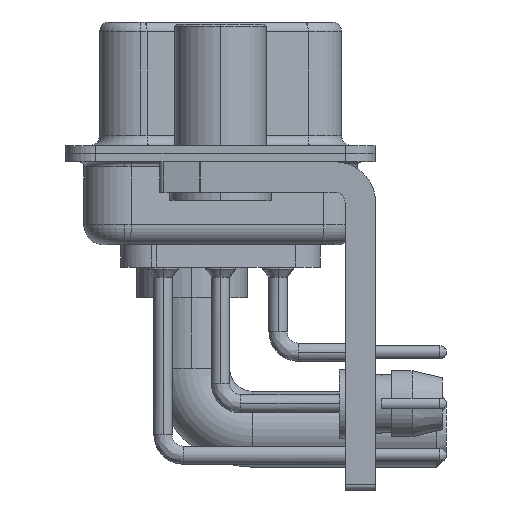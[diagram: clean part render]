
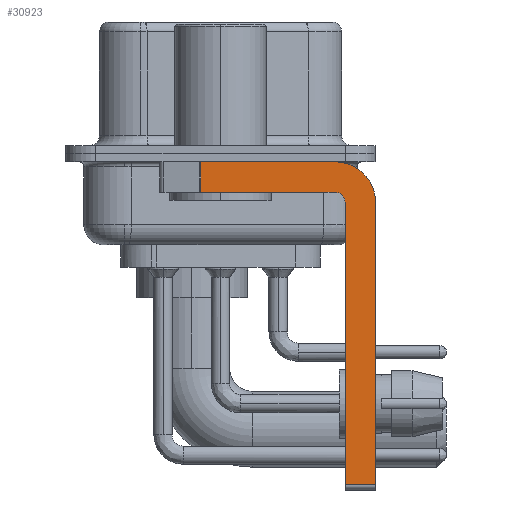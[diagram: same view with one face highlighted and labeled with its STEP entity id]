
A CAD part, left-side view. The second image highlights one B-rep face of the part: STEP entity #30923.
In plain terms, the highlighted planar face has unit normal (-1, 0, 0).
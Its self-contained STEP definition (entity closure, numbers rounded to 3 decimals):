
#96 = AXIS2_PLACEMENT_3D ( 'NONE', #14700, #20282, #21100 ) ;
#1183 = CARTESIAN_POINT ( 'NONE',  ( -2.9, 3., -0.4 ) ) ;
#1696 = VECTOR ( 'NONE', #13907, 1000. ) ;
#1845 = LINE ( 'NONE', #11345, #6708 ) ;
#3026 = DIRECTION ( 'NONE',  ( 0., 0., 1. ) ) ;
#3221 = CARTESIAN_POINT ( 'NONE',  ( -2.9, -7.65, -2.4 ) ) ;
#3273 = CARTESIAN_POINT ( 'NONE',  ( -2.9, -5.65, -2.4 ) ) ;
#3668 = ORIENTED_EDGE ( 'NONE', *, *, #4873, .T. ) ;
#4873 = EDGE_CURVE ( 'NONE', #5957, #13016, #1845, .T. ) ;
#4995 = CARTESIAN_POINT ( 'NONE',  ( -2.9, 0.978, -1.9 ) ) ;
#5515 = EDGE_CURVE ( 'NONE', #15541, #10681, #18696, .T. ) ;
#5957 = VERTEX_POINT ( 'NONE', #21525 ) ;
#6576 = EDGE_CURVE ( 'NONE', #24902, #39361, #7329, .T. ) ;
#6708 = VECTOR ( 'NONE', #36830, 1000. ) ;
#7329 = LINE ( 'NONE', #3221, #15511 ) ;
#7722 = LINE ( 'NONE', #23409, #1696 ) ;
#9892 = DIRECTION ( 'NONE',  ( 0., -1., 0. ) ) ;
#10085 = ORIENTED_EDGE ( 'NONE', *, *, #16367, .T. ) ;
#10681 = VERTEX_POINT ( 'NONE', #37434 ) ;
#11345 = CARTESIAN_POINT ( 'NONE',  ( -2.9, 0.978, -1.9 ) ) ;
#12985 = PLANE ( 'NONE',  #29920 ) ;
#13016 = VERTEX_POINT ( 'NONE', #4995 ) ;
#13907 = DIRECTION ( 'NONE',  ( 0., 1., 0. ) ) ;
#14700 = CARTESIAN_POINT ( 'NONE',  ( -2.9, -5.65, -2.4 ) ) ;
#15511 = VECTOR ( 'NONE', #15803, 1000. ) ;
#15541 = VERTEX_POINT ( 'NONE', #18514 ) ;
#15609 = ORIENTED_EDGE ( 'NONE', *, *, #5515, .F. ) ;
#15803 = DIRECTION ( 'NONE',  ( 0., 0., -1. ) ) ;
#16085 = VECTOR ( 'NONE', #3026, 1000. ) ;
#16202 = EDGE_CURVE ( 'NONE', #10681, #21532, #26743, .T. ) ;
#16367 = EDGE_CURVE ( 'NONE', #15541, #39361, #24037, .T. ) ;
#16476 = FACE_OUTER_BOUND ( 'NONE', #18847, .T. ) ;
#18172 = CARTESIAN_POINT ( 'NONE',  ( -2.9, -5.65, -0.4 ) ) ;
#18514 = CARTESIAN_POINT ( 'NONE',  ( -2.9, -6.15, -16.35 ) ) ;
#18696 = LINE ( 'NONE', #31349, #16085 ) ;
#18847 = EDGE_LOOP ( 'NONE', ( #21902, #3668, #19758, #30203, #15609, #10085, #38319, #26120 ) ) ;
#19758 = ORIENTED_EDGE ( 'NONE', *, *, #38857, .F. ) ;
#20282 = DIRECTION ( 'NONE',  ( 1., 0., 0. ) ) ;
#21100 = DIRECTION ( 'NONE',  ( 0., 0., -1. ) ) ;
#21521 = VERTEX_POINT ( 'NONE', #18172 ) ;
#21525 = CARTESIAN_POINT ( 'NONE',  ( -2.9, 0.978, -0.4 ) ) ;
#21532 = VERTEX_POINT ( 'NONE', #24800 ) ;
#21902 = ORIENTED_EDGE ( 'NONE', *, *, #35999, .F. ) ;
#22069 = AXIS2_PLACEMENT_3D ( 'NONE', #33155, #26322, #36080 ) ;
#23289 = DIRECTION ( 'NONE',  ( 0., -1., 0. ) ) ;
#23401 = VECTOR ( 'NONE', #9892, 1000. ) ;
#23409 = CARTESIAN_POINT ( 'NONE',  ( -2.9, -5.65, -1.9 ) ) ;
#23917 = EDGE_CURVE ( 'NONE', #21521, #24902, #26526, .T. ) ;
#24037 = LINE ( 'NONE', #36699, #23401 ) ;
#24800 = CARTESIAN_POINT ( 'NONE',  ( -2.9, -5.65, -1.9 ) ) ;
#24902 = VERTEX_POINT ( 'NONE', #36783 ) ;
#26120 = ORIENTED_EDGE ( 'NONE', *, *, #23917, .F. ) ;
#26279 = CARTESIAN_POINT ( 'NONE',  ( -2.9, -7.65, -16.35 ) ) ;
#26322 = DIRECTION ( 'NONE',  ( -1., 0., 0. ) ) ;
#26526 = CIRCLE ( 'NONE', #96, 2. ) ;
#26743 = CIRCLE ( 'NONE', #22069, 0.5 ) ;
#26853 = LINE ( 'NONE', #1183, #27348 ) ;
#27348 = VECTOR ( 'NONE', #23289, 1000. ) ;
#28294 = DIRECTION ( 'NONE',  ( 1., 0., 0. ) ) ;
#29920 = AXIS2_PLACEMENT_3D ( 'NONE', #3273, #28294, #35335 ) ;
#30203 = ORIENTED_EDGE ( 'NONE', *, *, #16202, .F. ) ;
#30923 = ADVANCED_FACE ( 'NONE', ( #16476 ), #12985, .F. ) ;
#31349 = CARTESIAN_POINT ( 'NONE',  ( -2.9, -6.15, -16.6 ) ) ;
#33155 = CARTESIAN_POINT ( 'NONE',  ( -2.9, -5.65, -2.4 ) ) ;
#35335 = DIRECTION ( 'NONE',  ( 0., 0., -1. ) ) ;
#35999 = EDGE_CURVE ( 'NONE', #5957, #21521, #26853, .T. ) ;
#36080 = DIRECTION ( 'NONE',  ( 0., 0., 1. ) ) ;
#36699 = CARTESIAN_POINT ( 'NONE',  ( -2.9, -5.65, -16.35 ) ) ;
#36783 = CARTESIAN_POINT ( 'NONE',  ( -2.9, -7.65, -2.4 ) ) ;
#36830 = DIRECTION ( 'NONE',  ( 0., 0., -1. ) ) ;
#37434 = CARTESIAN_POINT ( 'NONE',  ( -2.9, -6.15, -2.4 ) ) ;
#38319 = ORIENTED_EDGE ( 'NONE', *, *, #6576, .F. ) ;
#38857 = EDGE_CURVE ( 'NONE', #21532, #13016, #7722, .T. ) ;
#39361 = VERTEX_POINT ( 'NONE', #26279 ) ;
